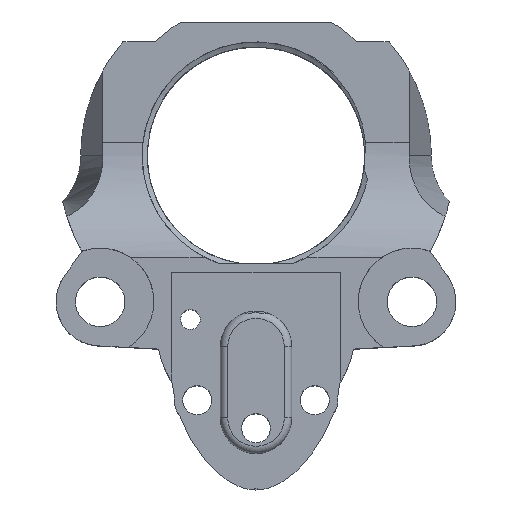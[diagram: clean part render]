
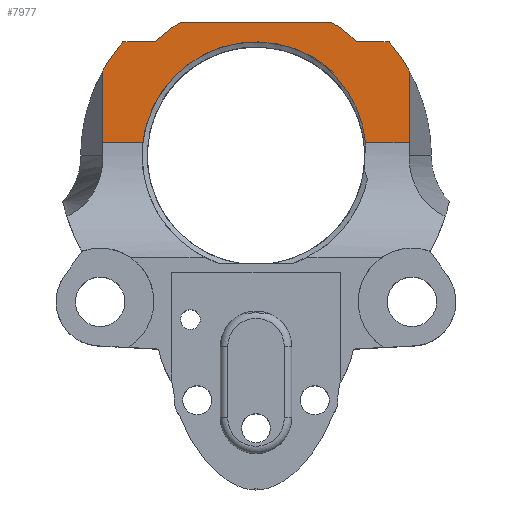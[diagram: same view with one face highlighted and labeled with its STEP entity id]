
A CAD part, top view. The second image highlights one B-rep face of the part: STEP entity #7977.
In plain terms, the highlighted planar face has unit normal (0, 0, 1).
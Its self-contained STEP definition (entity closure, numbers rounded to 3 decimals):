
#75 = PLANE ( 'NONE',  #7605 ) ;
#181 = VERTEX_POINT ( 'NONE', #9131 ) ;
#300 = DIRECTION ( 'NONE',  ( -1., 0., 0. ) ) ;
#394 = VERTEX_POINT ( 'NONE', #3717 ) ;
#732 = DIRECTION ( 'NONE',  ( 0., 0., 1. ) ) ;
#763 = AXIS2_PLACEMENT_3D ( 'NONE', #1420, #8057, #300 ) ;
#1040 = DIRECTION ( 'NONE',  ( 0., 0., -1. ) ) ;
#1163 = LINE ( 'NONE', #10783, #13206 ) ;
#1252 = CARTESIAN_POINT ( 'NONE',  ( 21.574, 61.688, -27.602 ) ) ;
#1386 = CARTESIAN_POINT ( 'NONE',  ( -6.622, 65.601, -27.602 ) ) ;
#1420 = CARTESIAN_POINT ( 'NONE',  ( 11.5, 50.101, -27.602 ) ) ;
#1548 = EDGE_CURVE ( 'NONE', #11715, #2960, #4063, .T. ) ;
#1743 = DIRECTION ( 'NONE',  ( 1., 0., 0. ) ) ;
#1767 = ORIENTED_EDGE ( 'NONE', *, *, #1845, .T. ) ;
#1779 = ORIENTED_EDGE ( 'NONE', *, *, #10953, .T. ) ;
#1845 = EDGE_CURVE ( 'NONE', #394, #5244, #9196, .T. ) ;
#1849 = VECTOR ( 'NONE', #11603, 1000. ) ;
#1865 = VERTEX_POINT ( 'NONE', #4505 ) ;
#1944 = ORIENTED_EDGE ( 'NONE', *, *, #13991, .T. ) ;
#1996 = CARTESIAN_POINT ( 'NONE',  ( 25.201, 56.596, -27.602 ) ) ;
#2224 = CARTESIAN_POINT ( 'NONE',  ( 18.13, 64.083, -27.602 ) ) ;
#2244 = LINE ( 'NONE', #12305, #5514 ) ;
#2325 = AXIS2_PLACEMENT_3D ( 'NONE', #10444, #12669, #2793 ) ;
#2365 = EDGE_CURVE ( 'NONE', #1865, #13029, #13841, .T. ) ;
#2426 = ORIENTED_EDGE ( 'NONE', *, *, #10675, .T. ) ;
#2620 = CARTESIAN_POINT ( 'NONE',  ( 11.5, 50.101, -27.602 ) ) ;
#2793 = DIRECTION ( 'NONE',  ( -1., 0., 0. ) ) ;
#2834 = CARTESIAN_POINT ( 'NONE',  ( -46., 51.886, -27.602 ) ) ;
#2960 = VERTEX_POINT ( 'NONE', #4053 ) ;
#3106 = CARTESIAN_POINT ( 'NONE',  ( 23.845, 59.032, -27.602 ) ) ;
#3136 = DIRECTION ( 'NONE',  ( -1., 0., 0. ) ) ;
#3138 = EDGE_CURVE ( 'NONE', #7957, #4729, #9011, .T. ) ;
#3296 = CARTESIAN_POINT ( 'NONE',  ( 26.22, 53.28, -27.602 ) ) ;
#3394 = DIRECTION ( 'NONE',  ( 1., 0., 0. ) ) ;
#3425 = CARTESIAN_POINT ( 'NONE',  ( 23.017, 60.16, -27.602 ) ) ;
#3468 = CARTESIAN_POINT ( 'NONE',  ( 17.5, 64.387, -27.602 ) ) ;
#3476 = ORIENTED_EDGE ( 'NONE', *, *, #5607, .F. ) ;
#3568 = CARTESIAN_POINT ( 'NONE',  ( 32.367, 61.643, -27.602 ) ) ;
#3702 = CIRCLE ( 'NONE', #12507, 20. ) ;
#3717 = CARTESIAN_POINT ( 'NONE',  ( -2.275, 65.601, -27.602 ) ) ;
#3737 = DIRECTION ( 'NONE',  ( -1., 0., 0. ) ) ;
#3768 = CARTESIAN_POINT ( 'NONE',  ( -3.897, 51.886, -27.602 ) ) ;
#3856 = ORIENTED_EDGE ( 'NONE', *, *, #11070, .T. ) ;
#3977 = DIRECTION ( 'NONE',  ( 0., 1., 0. ) ) ;
#4053 = CARTESIAN_POINT ( 'NONE',  ( 29.622, 65.601, -27.602 ) ) ;
#4063 = CIRCLE ( 'NONE', #5994, 23.846 ) ;
#4399 = AXIS2_PLACEMENT_3D ( 'NONE', #10646, #732, #5150 ) ;
#4441 = LINE ( 'NONE', #2834, #1849 ) ;
#4504 = EDGE_CURVE ( 'NONE', #9721, #11715, #2244, .T. ) ;
#4505 = CARTESIAN_POINT ( 'NONE',  ( 21.685, 68.313, -27.602 ) ) ;
#4532 = EDGE_CURVE ( 'NONE', #11955, #1865, #12391, .T. ) ;
#4573 = CARTESIAN_POINT ( 'NONE',  ( 19.933, 63.003, -27.602 ) ) ;
#4729 = VERTEX_POINT ( 'NONE', #6009 ) ;
#5051 = EDGE_CURVE ( 'NONE', #9844, #181, #7323, .T. ) ;
#5070 = ORIENTED_EDGE ( 'NONE', *, *, #4504, .T. ) ;
#5150 = DIRECTION ( 'NONE',  ( -1., 0., 0. ) ) ;
#5244 = VERTEX_POINT ( 'NONE', #1386 ) ;
#5264 = CARTESIAN_POINT ( 'NONE',  ( 25.697, 55.304, -27.602 ) ) ;
#5447 = CARTESIAN_POINT ( 'NONE',  ( 1.315, 68.313, -27.602 ) ) ;
#5501 = CARTESIAN_POINT ( 'NONE',  ( -9.367, 68.313, -27.602 ) ) ;
#5514 = VECTOR ( 'NONE', #3977, 1000. ) ;
#5607 = EDGE_CURVE ( 'NONE', #181, #7120, #6548, .T. ) ;
#5634 = CARTESIAN_POINT ( 'NONE',  ( 11.5, 51.101, -27.602 ) ) ;
#5994 = AXIS2_PLACEMENT_3D ( 'NONE', #2620, #11592, #3737 ) ;
#6009 = CARTESIAN_POINT ( 'NONE',  ( -9.367, 51.886, -27.602 ) ) ;
#6548 = CIRCLE ( 'NONE', #763, 15.5 ) ;
#6582 = DIRECTION ( 'NONE',  ( -1., 0., 0. ) ) ;
#6617 = DIRECTION ( 'NONE',  ( 0., -1., 0. ) ) ;
#7034 = CARTESIAN_POINT ( 'NONE',  ( 32.367, 51.886, -27.602 ) ) ;
#7120 = VERTEX_POINT ( 'NONE', #3768 ) ;
#7323 = B_SPLINE_CURVE_WITH_KNOTS ( 'NONE', 3,
 ( #9886, #14118, #3296, #8587, #5264, #1996, #10795, #9749, #9704, #3106, #11073, #3425, #13280, #1252, #12268, #4573, #11204, #2224, #3468, #10102 ),
 .UNSPECIFIED., .F., .F.,
 ( 4, 2, 2, 2, 2, 2, 2, 2, 2, 4 ),
 ( 0., 0.002, 0.004, 0.006, 0.007, 0.008, 0.011, 0.013, 0.015, 0.017 ),
 .UNSPECIFIED. ) ;
#7605 = AXIS2_PLACEMENT_3D ( 'NONE', #11061, #9967, #7751 ) ;
#7751 = DIRECTION ( 'NONE',  ( -1., 0., 0. ) ) ;
#7774 = CARTESIAN_POINT ( 'NONE',  ( -46., 51.886, -27.602 ) ) ;
#7957 = VERTEX_POINT ( 'NONE', #9872 ) ;
#7977 = ADVANCED_FACE ( 'NONE', ( #10998 ), #75, .F. ) ;
#8041 = ORIENTED_EDGE ( 'NONE', *, *, #3138, .T. ) ;
#8057 = DIRECTION ( 'NONE',  ( 0., 0., 1. ) ) ;
#8587 = CARTESIAN_POINT ( 'NONE',  ( 25.902, 54.641, -27.602 ) ) ;
#8692 = ORIENTED_EDGE ( 'NONE', *, *, #4532, .F. ) ;
#8879 = VECTOR ( 'NONE', #10164, 1000. ) ;
#9011 = LINE ( 'NONE', #5501, #11963 ) ;
#9131 = CARTESIAN_POINT ( 'NONE',  ( 16.848, 64.649, -27.602 ) ) ;
#9196 = LINE ( 'NONE', #14280, #8879 ) ;
#9704 = CARTESIAN_POINT ( 'NONE',  ( 24.224, 58.444, -27.602 ) ) ;
#9721 = VERTEX_POINT ( 'NONE', #7034 ) ;
#9749 = CARTESIAN_POINT ( 'NONE',  ( 24.404, 58.142, -27.602 ) ) ;
#9844 = VERTEX_POINT ( 'NONE', #12448 ) ;
#9872 = CARTESIAN_POINT ( 'NONE',  ( -9.367, 61.643, -27.602 ) ) ;
#9886 = CARTESIAN_POINT ( 'NONE',  ( 26.396, 51.886, -27.602 ) ) ;
#9967 = DIRECTION ( 'NONE',  ( 0., 0., -1. ) ) ;
#10102 = CARTESIAN_POINT ( 'NONE',  ( 16.848, 64.649, -27.602 ) ) ;
#10164 = DIRECTION ( 'NONE',  ( -1., 0., 0. ) ) ;
#10444 = CARTESIAN_POINT ( 'NONE',  ( 11.5, 51.101, -27.602 ) ) ;
#10589 = ORIENTED_EDGE ( 'NONE', *, *, #5051, .F. ) ;
#10646 = CARTESIAN_POINT ( 'NONE',  ( 11.5, 50.101, -27.602 ) ) ;
#10675 = EDGE_CURVE ( 'NONE', #5244, #7957, #12191, .T. ) ;
#10783 = CARTESIAN_POINT ( 'NONE',  ( 31.189, 65.601, -27.602 ) ) ;
#10795 = CARTESIAN_POINT ( 'NONE',  ( 24.91, 57.225, -27.602 ) ) ;
#10873 = ORIENTED_EDGE ( 'NONE', *, *, #14014, .F. ) ;
#10953 = EDGE_CURVE ( 'NONE', #4729, #7120, #4441, .T. ) ;
#10998 = FACE_OUTER_BOUND ( 'NONE', #12115, .T. ) ;
#11061 = CARTESIAN_POINT ( 'NONE',  ( -46., 68.313, -27.602 ) ) ;
#11070 = EDGE_CURVE ( 'NONE', #2960, #13029, #1163, .T. ) ;
#11073 = CARTESIAN_POINT ( 'NONE',  ( 23.645, 59.319, -27.602 ) ) ;
#11204 = CARTESIAN_POINT ( 'NONE',  ( 19.348, 63.39, -27.602 ) ) ;
#11592 = DIRECTION ( 'NONE',  ( 0., 0., 1. ) ) ;
#11603 = DIRECTION ( 'NONE',  ( 1., 0., 0. ) ) ;
#11715 = VERTEX_POINT ( 'NONE', #3568 ) ;
#11822 = LINE ( 'NONE', #7774, #14048 ) ;
#11955 = VERTEX_POINT ( 'NONE', #5447 ) ;
#11963 = VECTOR ( 'NONE', #6617, 1000. ) ;
#12115 = EDGE_LOOP ( 'NONE', ( #5070, #13822, #3856, #12632, #8692, #10873, #1767, #2426, #8041, #1779, #3476, #10589, #1944 ) ) ;
#12191 = CIRCLE ( 'NONE', #4399, 23.846 ) ;
#12268 = CARTESIAN_POINT ( 'NONE',  ( 21.046, 62.152, -27.602 ) ) ;
#12305 = CARTESIAN_POINT ( 'NONE',  ( 32.367, 68.315, -27.602 ) ) ;
#12391 = LINE ( 'NONE', #13766, #13419 ) ;
#12448 = CARTESIAN_POINT ( 'NONE',  ( 26.396, 51.886, -27.602 ) ) ;
#12507 = AXIS2_PLACEMENT_3D ( 'NONE', #5634, #1040, #6582 ) ;
#12632 = ORIENTED_EDGE ( 'NONE', *, *, #2365, .F. ) ;
#12669 = DIRECTION ( 'NONE',  ( 0., 0., -1. ) ) ;
#12992 = CARTESIAN_POINT ( 'NONE',  ( 25.275, 65.601, -27.602 ) ) ;
#13029 = VERTEX_POINT ( 'NONE', #12992 ) ;
#13206 = VECTOR ( 'NONE', #3136, 1000. ) ;
#13280 = CARTESIAN_POINT ( 'NONE',  ( 22.557, 60.693, -27.602 ) ) ;
#13419 = VECTOR ( 'NONE', #1743, 1000. ) ;
#13766 = CARTESIAN_POINT ( 'NONE',  ( 24.914, 68.313, -27.602 ) ) ;
#13822 = ORIENTED_EDGE ( 'NONE', *, *, #1548, .T. ) ;
#13841 = CIRCLE ( 'NONE', #2325, 20. ) ;
#13991 = EDGE_CURVE ( 'NONE', #9844, #9721, #11822, .T. ) ;
#14014 = EDGE_CURVE ( 'NONE', #394, #11955, #3702, .T. ) ;
#14048 = VECTOR ( 'NONE', #3394, 1000. ) ;
#14118 = CARTESIAN_POINT ( 'NONE',  ( 26.333, 52.585, -27.602 ) ) ;
#14280 = CARTESIAN_POINT ( 'NONE',  ( -2.275, 65.601, -27.602 ) ) ;
